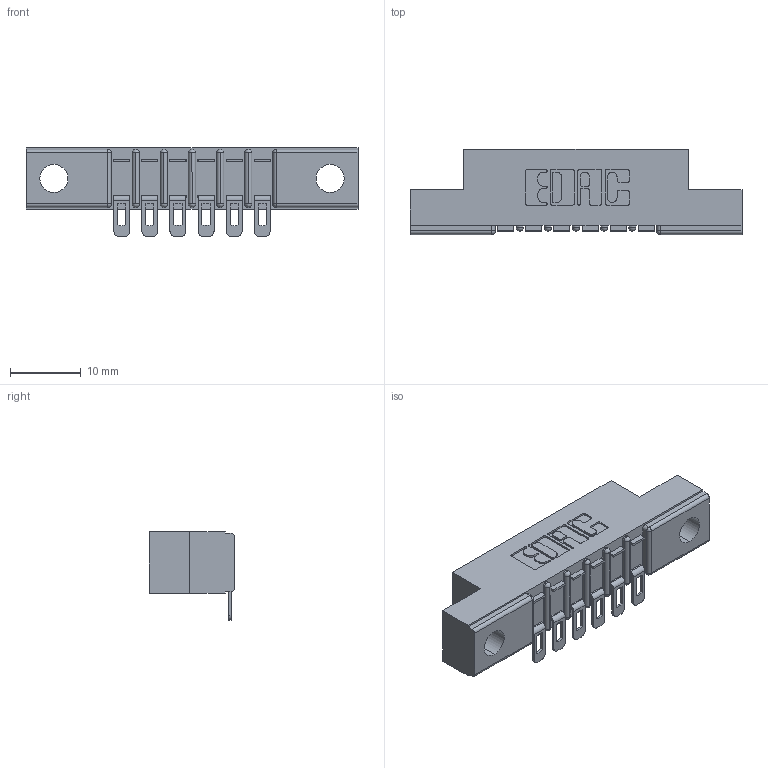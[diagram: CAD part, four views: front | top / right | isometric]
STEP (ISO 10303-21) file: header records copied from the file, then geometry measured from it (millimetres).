
FILE_DESCRIPTION (( 'STEP AP203' ), '1' );
FILE_NAME ('357-006-554-102.STEP', '2019-09-16T17:07:41', ( '' ), ( '' ), 'SwSTEP 2.0', 'SolidWorks 2016', '' );
FILE_SCHEMA (( 'CONFIG_CONTROL_DESIGN' ));
Length unit declared in the file: inch
Products named in the file (3): 307 Part_.128 Dia Mounting Holes; 307-290-002_554; 357-006-554-102
Assembly tree (7 placements, depth 2):
  357-006-554-102
    307 Part_.128 Dia Mounting Holes
    307-290-002_554  x6
Bounding box: 46.79 x 12.01 x 12.52 mm (x, y, z)
Volume: 2994.7 mm3; surface area: 4430.1 mm2
Topology: 7 solids, 7 shells, 611 faces, 1841 edges, 1206 vertices
Faces by surface type: plane 346, cylinder 251, sphere 14
Entity records: 10549 total; most frequent: CARTESIAN_POINT 1774, ORIENTED_EDGE 1764, DIRECTION 1746, EDGE_CURVE 882, VECTOR 650, LINE 650, VERTEX_POINT 576, AXIS2_PLACEMENT_3D 548
